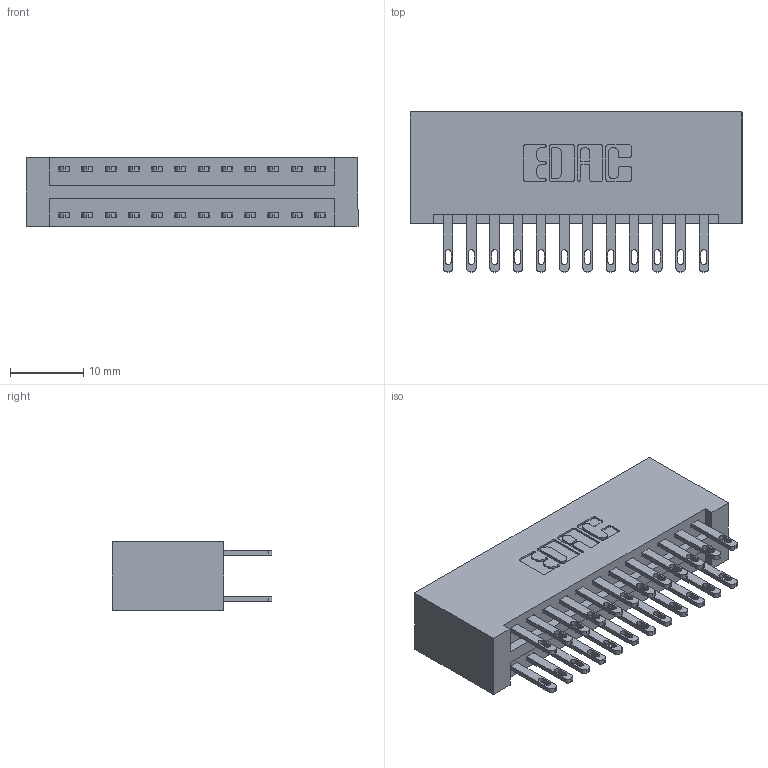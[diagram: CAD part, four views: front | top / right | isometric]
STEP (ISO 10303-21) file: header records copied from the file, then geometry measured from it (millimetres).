
FILE_DESCRIPTION (( 'STEP AP203' ), '1' );
FILE_NAME ('896-024-500-201.STEP', '2021-07-27T17:19:45', ( '' ), ( '' ), 'SwSTEP 2.0', 'SolidWorks 2020', '' );
FILE_SCHEMA (( 'CONFIG_CONTROL_DESIGN' ));
Length unit declared in the file: inch
Products named in the file (3): 345-292-001_345-293-100; 846 Part_No Mounting Lugs; 896-024-500-201
Assembly tree (25 placements, depth 2):
  896-024-500-201
    846 Part_No Mounting Lugs
    345-292-001_345-293-100  x24
Bounding box: 45.34 x 21.84 x 9.4 mm (x, y, z)
Volume: 4834.7 mm3; surface area: 6588.5 mm2
Topology: 25 solids, 25 shells, 1266 faces, 3833 edges, 2554 vertices
Faces by surface type: plane 768, cylinder 498
Entity records: 11523 total; most frequent: CARTESIAN_POINT 1936, ORIENTED_EDGE 1870, DIRECTION 1755, EDGE_CURVE 935, VECTOR 759, LINE 759, VERTEX_POINT 622, AXIS2_PLACEMENT_3D 498
